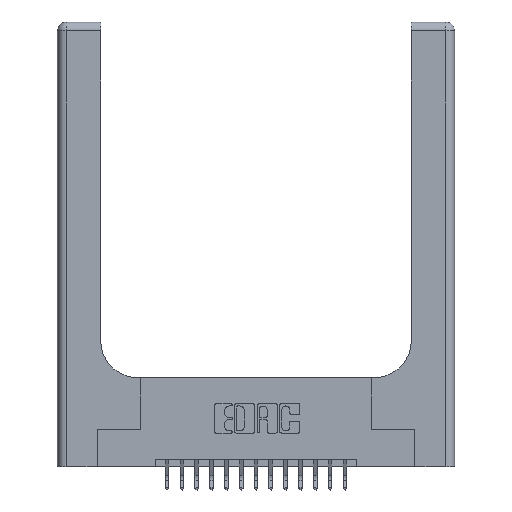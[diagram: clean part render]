
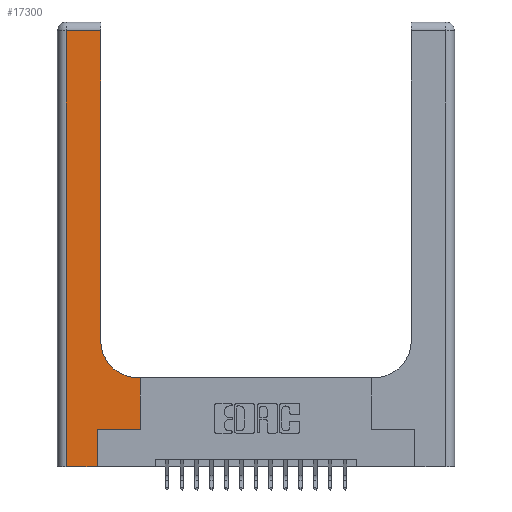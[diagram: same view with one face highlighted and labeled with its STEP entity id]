
A CAD part, top view. The second image highlights one B-rep face of the part: STEP entity #17300.
In plain terms, the highlighted planar face has unit normal (0, 0, 1).
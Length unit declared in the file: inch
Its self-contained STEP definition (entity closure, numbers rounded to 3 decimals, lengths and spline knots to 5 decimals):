
#603 = VECTOR ( 'NONE', #6737, 39.37008 ) ;
#798 = CARTESIAN_POINT ( 'NONE',  ( 0.5585, 0.25, 0.37 ) ) ;
#845 = EDGE_CURVE ( 'NONE', #10163, #6476, #2445, .T. ) ;
#951 = VECTOR ( 'NONE', #6132, 39.37008 ) ;
#1276 = CARTESIAN_POINT ( 'NONE',  ( 0.269, 0.25, 0.37 ) ) ;
#1869 = CARTESIAN_POINT ( 'NONE',  ( 0.5415, 0.85, 0.37 ) ) ;
#2193 = CIRCLE ( 'NONE', #10506, 0.25 ) ;
#2445 = LINE ( 'NONE', #10995, #5978 ) ;
#2550 = DIRECTION ( 'NONE',  ( 0., 1., 0. ) ) ;
#2876 = VERTEX_POINT ( 'NONE', #4101 ) ;
#3009 = VECTOR ( 'NONE', #2550, 39.37008 ) ;
#3037 = ORIENTED_EDGE ( 'NONE', *, *, #4293, .T. ) ;
#3158 = VERTEX_POINT ( 'NONE', #9356 ) ;
#3365 = ORIENTED_EDGE ( 'NONE', *, *, #16810, .T. ) ;
#3575 = DIRECTION ( 'NONE',  ( 0., -1., 0. ) ) ;
#3996 = VERTEX_POINT ( 'NONE', #14729 ) ;
#4101 = CARTESIAN_POINT ( 'NONE',  ( 0.269, 0., 0.37 ) ) ;
#4293 = EDGE_CURVE ( 'NONE', #11530, #18459, #8854, .T. ) ;
#5194 = VECTOR ( 'NONE', #6520, 39.37008 ) ;
#5320 = LINE ( 'NONE', #11135, #11433 ) ;
#5633 = CARTESIAN_POINT ( 'NONE',  ( 0.5415, 0.6, 0.37 ) ) ;
#5719 = EDGE_LOOP ( 'NONE', ( #11286, #6138, #3365, #11320, #11338, #3037, #17369, #13957, #16919 ) ) ;
#5978 = VECTOR ( 'NONE', #8059, 39.37008 ) ;
#6010 = CARTESIAN_POINT ( 'NONE',  ( 0.06, 2.94, 0.37 ) ) ;
#6132 = DIRECTION ( 'NONE',  ( -1., 0., 0. ) ) ;
#6138 = ORIENTED_EDGE ( 'NONE', *, *, #845, .T. ) ;
#6250 = VECTOR ( 'NONE', #13748, 39.37008 ) ;
#6409 = DIRECTION ( 'NONE',  ( 0., 0., -1. ) ) ;
#6476 = VERTEX_POINT ( 'NONE', #6010 ) ;
#6520 = DIRECTION ( 'NONE',  ( 0., 1., 0. ) ) ;
#6712 = CARTESIAN_POINT ( 'NONE',  ( 0.2915, 3., 0.37 ) ) ;
#6717 = EDGE_CURVE ( 'NONE', #2876, #11530, #9612, .T. ) ;
#6737 = DIRECTION ( 'NONE',  ( 1., 0., 0. ) ) ;
#6921 = DIRECTION ( 'NONE',  ( 1., 0., 0. ) ) ;
#7099 = AXIS2_PLACEMENT_3D ( 'NONE', #7924, #15661, #14389 ) ;
#7286 = LINE ( 'NONE', #19439, #951 ) ;
#7924 = CARTESIAN_POINT ( 'NONE',  ( 0., 3., 0.37 ) ) ;
#7972 = VERTEX_POINT ( 'NONE', #15346 ) ;
#8059 = DIRECTION ( 'NONE',  ( -1., 0., 0. ) ) ;
#8854 = LINE ( 'NONE', #15869, #603 ) ;
#9356 = CARTESIAN_POINT ( 'NONE',  ( 0.2915, 0.85, 0.37 ) ) ;
#9366 = DIRECTION ( 'NONE',  ( 1., 0., 0. ) ) ;
#9464 = CARTESIAN_POINT ( 'NONE',  ( 0.5585, 0.25, 0.37 ) ) ;
#9612 = LINE ( 'NONE', #16098, #3009 ) ;
#9814 = VERTEX_POINT ( 'NONE', #5633 ) ;
#10163 = VERTEX_POINT ( 'NONE', #11899 ) ;
#10502 = FACE_OUTER_BOUND ( 'NONE', #5719, .T. ) ;
#10506 = AXIS2_PLACEMENT_3D ( 'NONE', #1869, #6409, #9366 ) ;
#10608 = LINE ( 'NONE', #6712, #5194 ) ;
#10923 = PLANE ( 'NONE',  #7099 ) ;
#10995 = CARTESIAN_POINT ( 'NONE',  ( 0., 2.94, 0.37 ) ) ;
#11135 = CARTESIAN_POINT ( 'NONE',  ( 0.06, 3., 0.37 ) ) ;
#11141 = EDGE_CURVE ( 'NONE', #3158, #10163, #10608, .T. ) ;
#11286 = ORIENTED_EDGE ( 'NONE', *, *, #11141, .T. ) ;
#11320 = ORIENTED_EDGE ( 'NONE', *, *, #15390, .T. ) ;
#11338 = ORIENTED_EDGE ( 'NONE', *, *, #6717, .T. ) ;
#11433 = VECTOR ( 'NONE', #3575, 39.37008 ) ;
#11530 = VERTEX_POINT ( 'NONE', #1276 ) ;
#11899 = CARTESIAN_POINT ( 'NONE',  ( 0.2915, 2.94, 0.37 ) ) ;
#13077 = LINE ( 'NONE', #9464, #6250 ) ;
#13394 = EDGE_CURVE ( 'NONE', #3996, #9814, #7286, .T. ) ;
#13748 = DIRECTION ( 'NONE',  ( 0., 1., 0. ) ) ;
#13957 = ORIENTED_EDGE ( 'NONE', *, *, #13394, .T. ) ;
#14389 = DIRECTION ( 'NONE',  ( -1., 0., 0. ) ) ;
#14729 = CARTESIAN_POINT ( 'NONE',  ( 0.5585, 0.6, 0.37 ) ) ;
#14833 = VECTOR ( 'NONE', #6921, 39.37008 ) ;
#15346 = CARTESIAN_POINT ( 'NONE',  ( 0.06, 0., 0.37 ) ) ;
#15390 = EDGE_CURVE ( 'NONE', #7972, #2876, #18851, .T. ) ;
#15661 = DIRECTION ( 'NONE',  ( 0., 0., -1. ) ) ;
#15869 = CARTESIAN_POINT ( 'NONE',  ( 0.269, 0.25, 0.37 ) ) ;
#16098 = CARTESIAN_POINT ( 'NONE',  ( 0.269, 0., 0.37 ) ) ;
#16810 = EDGE_CURVE ( 'NONE', #6476, #7972, #5320, .T. ) ;
#16919 = ORIENTED_EDGE ( 'NONE', *, *, #19536, .T. ) ;
#17300 = ADVANCED_FACE ( 'NONE', ( #10502 ), #10923, .F. ) ;
#17361 = CARTESIAN_POINT ( 'NONE',  ( 0., 0., 0.37 ) ) ;
#17369 = ORIENTED_EDGE ( 'NONE', *, *, #18298, .T. ) ;
#18298 = EDGE_CURVE ( 'NONE', #18459, #3996, #13077, .T. ) ;
#18459 = VERTEX_POINT ( 'NONE', #798 ) ;
#18851 = LINE ( 'NONE', #17361, #14833 ) ;
#19439 = CARTESIAN_POINT ( 'NONE',  ( 0.2915, 0.6, 0.37 ) ) ;
#19536 = EDGE_CURVE ( 'NONE', #9814, #3158, #2193, .T. ) ;
